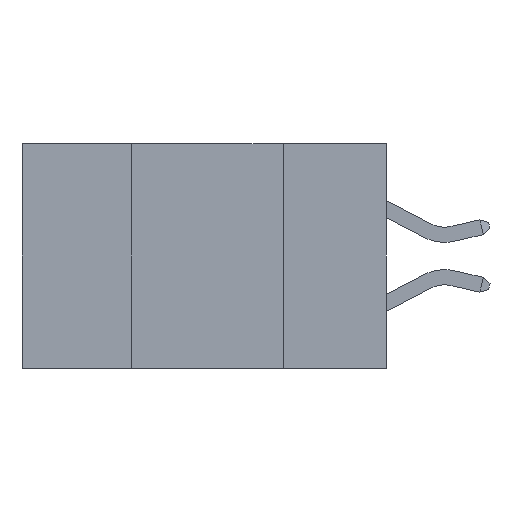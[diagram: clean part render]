
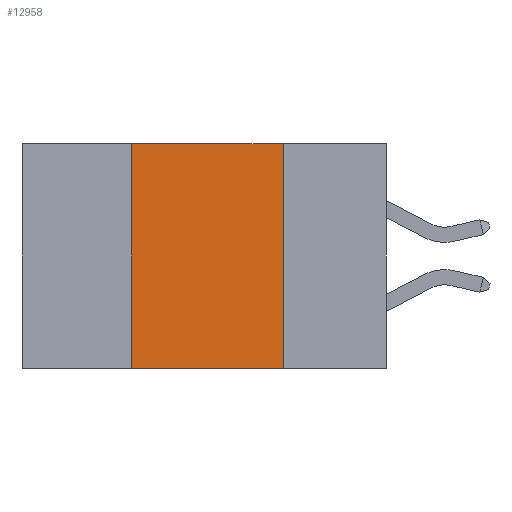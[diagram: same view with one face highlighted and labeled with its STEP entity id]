
A CAD part, left-side view. The second image highlights one B-rep face of the part: STEP entity #12958.
In plain terms, the highlighted planar face has unit normal (-1, 0, 0).
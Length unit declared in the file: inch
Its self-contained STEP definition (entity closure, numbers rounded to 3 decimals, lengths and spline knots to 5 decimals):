
#754 = DIRECTION ( 'NONE',  ( 0., 0., -1. ) ) ;
#1525 = LINE ( 'NONE', #4985, #9705 ) ;
#1885 = CARTESIAN_POINT ( 'NONE',  ( 0., 0.6, 0. ) ) ;
#2182 = EDGE_CURVE ( 'NONE', #3915, #11372, #7185, .T. ) ;
#2882 = ORIENTED_EDGE ( 'NONE', *, *, #2182, .T. ) ;
#3527 = AXIS2_PLACEMENT_3D ( 'NONE', #1885, #7255, #754 ) ;
#3529 = DIRECTION ( 'NONE',  ( 0., -1., 0. ) ) ;
#3915 = VERTEX_POINT ( 'NONE', #10452 ) ;
#4122 = VECTOR ( 'NONE', #4998, 39.37008 ) ;
#4440 = ORIENTED_EDGE ( 'NONE', *, *, #6366, .F. ) ;
#4474 = CARTESIAN_POINT ( 'NONE',  ( 0., 0.17, 0. ) ) ;
#4520 = ORIENTED_EDGE ( 'NONE', *, *, #5643, .F. ) ;
#4706 = VERTEX_POINT ( 'NONE', #4474 ) ;
#4964 = DIRECTION ( 'NONE',  ( 0., -1., 0. ) ) ;
#4985 = CARTESIAN_POINT ( 'NONE',  ( 0., 0.6, 0. ) ) ;
#4998 = DIRECTION ( 'NONE',  ( 0., 0., -1. ) ) ;
#5013 = CARTESIAN_POINT ( 'NONE',  ( 0., 0.6, -0.37 ) ) ;
#5048 = CARTESIAN_POINT ( 'NONE',  ( 0., 0.17, -0.37 ) ) ;
#5600 = FACE_OUTER_BOUND ( 'NONE', #9568, .T. ) ;
#5643 = EDGE_CURVE ( 'NONE', #3915, #13029, #8422, .T. ) ;
#6366 = EDGE_CURVE ( 'NONE', #13029, #4706, #1525, .T. ) ;
#7185 = LINE ( 'NONE', #5013, #9640 ) ;
#7255 = DIRECTION ( 'NONE',  ( 1., 0., 0. ) ) ;
#7440 = VECTOR ( 'NONE', #12718, 39.37008 ) ;
#8093 = CARTESIAN_POINT ( 'NONE',  ( 0., 0.17, -0.37 ) ) ;
#8422 = LINE ( 'NONE', #12763, #7440 ) ;
#8593 = ORIENTED_EDGE ( 'NONE', *, *, #11609, .F. ) ;
#9568 = EDGE_LOOP ( 'NONE', ( #8593, #4440, #4520, #2882 ) ) ;
#9640 = VECTOR ( 'NONE', #3529, 39.37008 ) ;
#9705 = VECTOR ( 'NONE', #4964, 39.37008 ) ;
#10452 = CARTESIAN_POINT ( 'NONE',  ( 0., 0.42, -0.37 ) ) ;
#11372 = VERTEX_POINT ( 'NONE', #8093 ) ;
#11386 = PLANE ( 'NONE',  #3527 ) ;
#11609 = EDGE_CURVE ( 'NONE', #4706, #11372, #12501, .T. ) ;
#12501 = LINE ( 'NONE', #5048, #4122 ) ;
#12718 = DIRECTION ( 'NONE',  ( 0., 0., 1. ) ) ;
#12763 = CARTESIAN_POINT ( 'NONE',  ( 0., 0.42, -0.37 ) ) ;
#12958 = ADVANCED_FACE ( 'NONE', ( #5600 ), #11386, .F. ) ;
#13029 = VERTEX_POINT ( 'NONE', #13488 ) ;
#13488 = CARTESIAN_POINT ( 'NONE',  ( 0., 0.42, 0. ) ) ;
